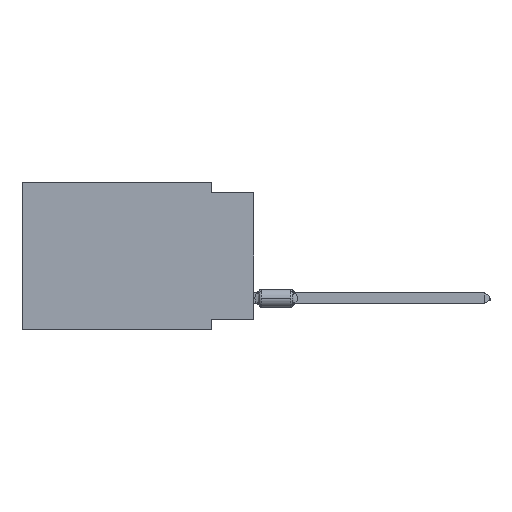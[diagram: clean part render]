
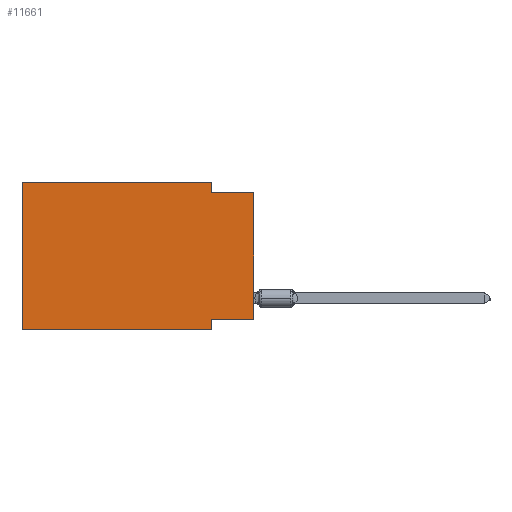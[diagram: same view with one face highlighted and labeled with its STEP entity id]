
A CAD part, left-side view. The second image highlights one B-rep face of the part: STEP entity #11661.
In plain terms, the highlighted planar face has unit normal (-1, 0, 0).
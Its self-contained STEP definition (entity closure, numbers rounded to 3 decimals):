
#496 = AXIS2_PLACEMENT_3D ( 'NONE', #1068, #41662, #2114 ) ;
#682 = EDGE_CURVE ( 'NONE', #45439, #26152, #18223, .T. ) ;
#1068 = CARTESIAN_POINT ( 'NONE',  ( 0., 13.97, 0. ) ) ;
#1090 = CARTESIAN_POINT ( 'NONE',  ( 0., 13.97, 0. ) ) ;
#2114 = DIRECTION ( 'NONE',  ( 0., 0., -1. ) ) ;
#2129 = DIRECTION ( 'NONE',  ( 0., 0., 1. ) ) ;
#4277 = EDGE_CURVE ( 'NONE', #38600, #12776, #6623, .T. ) ;
#5241 = LINE ( 'NONE', #13410, #32545 ) ;
#6623 = LINE ( 'NONE', #38767, #42978 ) ;
#8230 = EDGE_CURVE ( 'NONE', #26152, #28949, #33007, .T. ) ;
#10939 = DIRECTION ( 'NONE',  ( 0., -1., 0. ) ) ;
#11566 = CARTESIAN_POINT ( 'NONE',  ( 0., 0., -0.635 ) ) ;
#11661 = ADVANCED_FACE ( 'NONE', ( #17432 ), #37967, .F. ) ;
#12044 = EDGE_CURVE ( 'NONE', #45439, #33461, #5241, .T. ) ;
#12776 = VERTEX_POINT ( 'NONE', #11566 ) ;
#13410 = CARTESIAN_POINT ( 'NONE',  ( 0., 13.97, -8.89 ) ) ;
#13854 = EDGE_CURVE ( 'NONE', #28949, #22549, #50582, .T. ) ;
#14593 = CARTESIAN_POINT ( 'NONE',  ( 0., 0., -8.255 ) ) ;
#14765 = EDGE_LOOP ( 'NONE', ( #38622, #29041, #35345, #26486, #18576, #16237, #16745, #23364 ) ) ;
#16237 = ORIENTED_EDGE ( 'NONE', *, *, #12044, .T. ) ;
#16745 = ORIENTED_EDGE ( 'NONE', *, *, #35976, .F. ) ;
#17202 = VECTOR ( 'NONE', #25086, 1000. ) ;
#17432 = FACE_OUTER_BOUND ( 'NONE', #14765, .T. ) ;
#17949 = CARTESIAN_POINT ( 'NONE',  ( 0., 2.54, -8.89 ) ) ;
#18197 = EDGE_CURVE ( 'NONE', #38600, #24249, #30928, .T. ) ;
#18223 = LINE ( 'NONE', #42445, #27556 ) ;
#18576 = ORIENTED_EDGE ( 'NONE', *, *, #682, .F. ) ;
#19772 = VECTOR ( 'NONE', #30076, 1000. ) ;
#22098 = DIRECTION ( 'NONE',  ( 0., -1., 0. ) ) ;
#22170 = CARTESIAN_POINT ( 'NONE',  ( 0., 2.54, 0. ) ) ;
#22549 = VERTEX_POINT ( 'NONE', #23732 ) ;
#22639 = CARTESIAN_POINT ( 'NONE',  ( 0., 13.97, -8.89 ) ) ;
#23057 = CARTESIAN_POINT ( 'NONE',  ( 0., 0., -0.635 ) ) ;
#23364 = ORIENTED_EDGE ( 'NONE', *, *, #18197, .F. ) ;
#23732 = CARTESIAN_POINT ( 'NONE',  ( 0., 2.54, -0.635 ) ) ;
#24249 = VERTEX_POINT ( 'NONE', #28676 ) ;
#24366 = VECTOR ( 'NONE', #47221, 1000. ) ;
#25086 = DIRECTION ( 'NONE',  ( 0., -1., 0. ) ) ;
#26152 = VERTEX_POINT ( 'NONE', #38283 ) ;
#26486 = ORIENTED_EDGE ( 'NONE', *, *, #8230, .F. ) ;
#27556 = VECTOR ( 'NONE', #2129, 1000. ) ;
#28676 = CARTESIAN_POINT ( 'NONE',  ( 0., 2.54, -8.255 ) ) ;
#28949 = VERTEX_POINT ( 'NONE', #22170 ) ;
#29041 = ORIENTED_EDGE ( 'NONE', *, *, #50774, .F. ) ;
#30076 = DIRECTION ( 'NONE',  ( 0., 0., -1. ) ) ;
#30100 = LINE ( 'NONE', #45890, #49181 ) ;
#30928 = LINE ( 'NONE', #14593, #24366 ) ;
#32545 = VECTOR ( 'NONE', #22098, 1000. ) ;
#33007 = LINE ( 'NONE', #1090, #17202 ) ;
#33461 = VERTEX_POINT ( 'NONE', #17949 ) ;
#35345 = ORIENTED_EDGE ( 'NONE', *, *, #13854, .F. ) ;
#35976 = EDGE_CURVE ( 'NONE', #24249, #33461, #30100, .T. ) ;
#37967 = PLANE ( 'NONE',  #496 ) ;
#38283 = CARTESIAN_POINT ( 'NONE',  ( 0., 13.97, 0. ) ) ;
#38600 = VERTEX_POINT ( 'NONE', #42932 ) ;
#38622 = ORIENTED_EDGE ( 'NONE', *, *, #4277, .T. ) ;
#38767 = CARTESIAN_POINT ( 'NONE',  ( 0., 0., 0. ) ) ;
#41662 = DIRECTION ( 'NONE',  ( 1., 0., 0. ) ) ;
#42445 = CARTESIAN_POINT ( 'NONE',  ( 0., 13.97, 0. ) ) ;
#42932 = CARTESIAN_POINT ( 'NONE',  ( 0., 0., -8.255 ) ) ;
#42959 = DIRECTION ( 'NONE',  ( 0., 0., 1. ) ) ;
#42978 = VECTOR ( 'NONE', #42959, 1000. ) ;
#45439 = VERTEX_POINT ( 'NONE', #22639 ) ;
#45890 = CARTESIAN_POINT ( 'NONE',  ( 0., 2.54, -8.89 ) ) ;
#45912 = VECTOR ( 'NONE', #10939, 1000. ) ;
#47221 = DIRECTION ( 'NONE',  ( 0., 1., 0. ) ) ;
#47525 = LINE ( 'NONE', #23057, #45912 ) ;
#49181 = VECTOR ( 'NONE', #49572, 1000. ) ;
#49572 = DIRECTION ( 'NONE',  ( 0., 0., -1. ) ) ;
#50582 = LINE ( 'NONE', #50835, #19772 ) ;
#50774 = EDGE_CURVE ( 'NONE', #22549, #12776, #47525, .T. ) ;
#50835 = CARTESIAN_POINT ( 'NONE',  ( 0., 2.54, 0. ) ) ;
